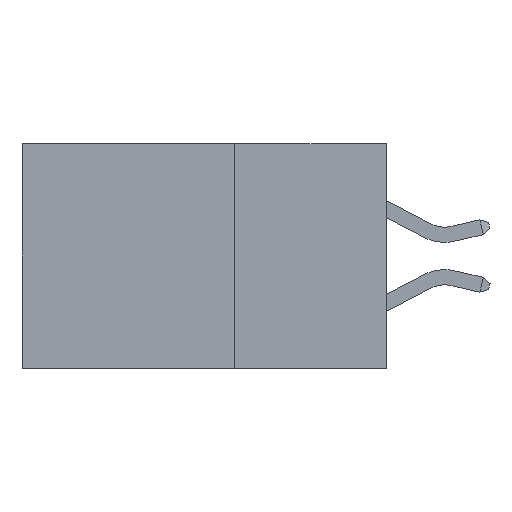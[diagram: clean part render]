
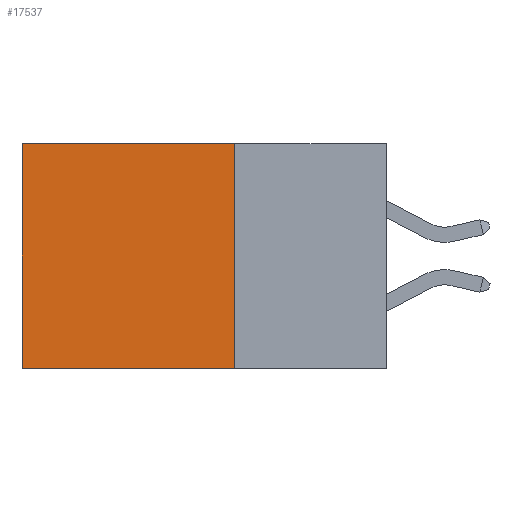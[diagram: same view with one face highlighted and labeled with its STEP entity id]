
A CAD part, left-side view. The second image highlights one B-rep face of the part: STEP entity #17537.
In plain terms, the highlighted planar face has unit normal (-1, 0, 0).
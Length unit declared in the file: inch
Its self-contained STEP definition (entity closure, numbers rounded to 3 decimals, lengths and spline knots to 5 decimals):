
#969 = DIRECTION ( 'NONE',  ( 0., 0., -1. ) ) ;
#2202 = CARTESIAN_POINT ( 'NONE',  ( 0.298, 0.25, 0. ) ) ;
#2927 = VECTOR ( 'NONE', #14190, 39.37008 ) ;
#2960 = VERTEX_POINT ( 'NONE', #13548 ) ;
#3742 = VECTOR ( 'NONE', #969, 39.37008 ) ;
#4147 = DIRECTION ( 'NONE',  ( 0., 1., 0. ) ) ;
#4305 = FACE_OUTER_BOUND ( 'NONE', #13779, .T. ) ;
#4582 = VECTOR ( 'NONE', #4147, 39.37008 ) ;
#5054 = LINE ( 'NONE', #13671, #3742 ) ;
#5920 = CARTESIAN_POINT ( 'NONE',  ( 0.298, 0.6, 0. ) ) ;
#7859 = DIRECTION ( 'NONE',  ( 0., 1., 0. ) ) ;
#7912 = VERTEX_POINT ( 'NONE', #5920 ) ;
#9943 = VERTEX_POINT ( 'NONE', #11502 ) ;
#11502 = CARTESIAN_POINT ( 'NONE',  ( 0.298, 0.6, -0.37 ) ) ;
#12596 = ORIENTED_EDGE ( 'NONE', *, *, #25930, .F. ) ;
#12764 = LINE ( 'NONE', #18099, #2927 ) ;
#13548 = CARTESIAN_POINT ( 'NONE',  ( 0.298, 0.25, 0. ) ) ;
#13665 = EDGE_CURVE ( 'NONE', #7912, #9943, #12764, .T. ) ;
#13671 = CARTESIAN_POINT ( 'NONE',  ( 0.298, 0.25, 0. ) ) ;
#13678 = EDGE_CURVE ( 'NONE', #2960, #7912, #16986, .T. ) ;
#13779 = EDGE_LOOP ( 'NONE', ( #19533, #23239, #12596, #21922 ) ) ;
#14190 = DIRECTION ( 'NONE',  ( 0., 0., -1. ) ) ;
#14379 = VECTOR ( 'NONE', #7859, 39.37008 ) ;
#14462 = AXIS2_PLACEMENT_3D ( 'NONE', #2202, #20888, #22944 ) ;
#14550 = PLANE ( 'NONE',  #14462 ) ;
#16287 = CARTESIAN_POINT ( 'NONE',  ( 0.298, 0.25, 0. ) ) ;
#16986 = LINE ( 'NONE', #16287, #14379 ) ;
#17537 = ADVANCED_FACE ( 'NONE', ( #4305 ), #14550, .F. ) ;
#17947 = VERTEX_POINT ( 'NONE', #19439 ) ;
#18099 = CARTESIAN_POINT ( 'NONE',  ( 0.298, 0.6, 0. ) ) ;
#18382 = EDGE_CURVE ( 'NONE', #17947, #9943, #20278, .T. ) ;
#19439 = CARTESIAN_POINT ( 'NONE',  ( 0.298, 0.25, -0.37 ) ) ;
#19533 = ORIENTED_EDGE ( 'NONE', *, *, #13665, .T. ) ;
#20278 = LINE ( 'NONE', #20772, #4582 ) ;
#20772 = CARTESIAN_POINT ( 'NONE',  ( 0.298, 0.25, -0.37 ) ) ;
#20888 = DIRECTION ( 'NONE',  ( 1., 0., 0. ) ) ;
#21922 = ORIENTED_EDGE ( 'NONE', *, *, #13678, .T. ) ;
#22944 = DIRECTION ( 'NONE',  ( 0., 0., -1. ) ) ;
#23239 = ORIENTED_EDGE ( 'NONE', *, *, #18382, .F. ) ;
#25930 = EDGE_CURVE ( 'NONE', #2960, #17947, #5054, .T. ) ;
